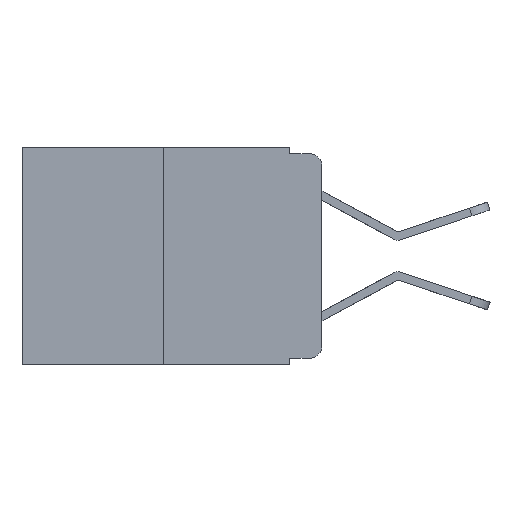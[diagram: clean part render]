
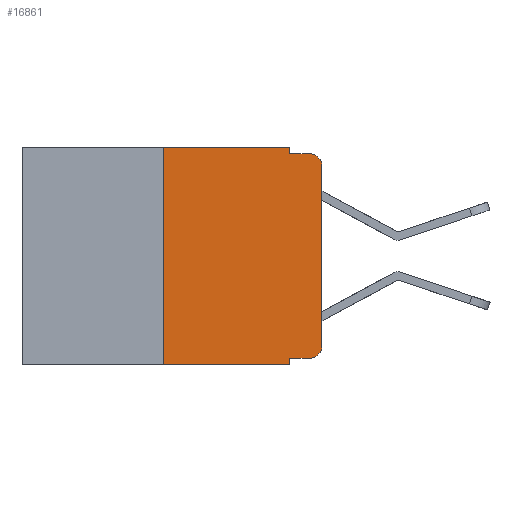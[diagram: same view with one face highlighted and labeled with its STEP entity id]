
A CAD part, left-side view. The second image highlights one B-rep face of the part: STEP entity #16861.
In plain terms, the highlighted planar face has unit normal (-1, 0, 0).
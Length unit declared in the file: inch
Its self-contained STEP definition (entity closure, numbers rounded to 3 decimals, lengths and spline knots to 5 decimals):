
#373 = DIRECTION ( 'NONE',  ( 0., 0., 1. ) ) ;
#494 = CARTESIAN_POINT ( 'NONE',  ( 0., 0.473, -0.343 ) ) ;
#852 = CARTESIAN_POINT ( 'NONE',  ( 0., 0.051, -0.01 ) ) ;
#1070 = EDGE_CURVE ( 'NONE', #14633, #12487, #20263, .T. ) ;
#1912 = LINE ( 'NONE', #2142, #10942 ) ;
#2142 = CARTESIAN_POINT ( 'NONE',  ( 0., 0.051, 0. ) ) ;
#2144 = CARTESIAN_POINT ( 'NONE',  ( 0., 0.25, -0.343 ) ) ;
#2176 = LINE ( 'NONE', #494, #15913 ) ;
#2320 = DIRECTION ( 'NONE',  ( 0., -1., 0. ) ) ;
#3552 = CARTESIAN_POINT ( 'NONE',  ( 0., 0.473, 0. ) ) ;
#3601 = ORIENTED_EDGE ( 'NONE', *, *, #10700, .F. ) ;
#3766 = EDGE_CURVE ( 'NONE', #4476, #6457, #15934, .T. ) ;
#4034 = CARTESIAN_POINT ( 'NONE',  ( 0., 0.02, -0.333 ) ) ;
#4049 = ORIENTED_EDGE ( 'NONE', *, *, #1070, .T. ) ;
#4253 = VERTEX_POINT ( 'NONE', #15675 ) ;
#4284 = LINE ( 'NONE', #21604, #13977 ) ;
#4476 = VERTEX_POINT ( 'NONE', #15097 ) ;
#5016 = VERTEX_POINT ( 'NONE', #8827 ) ;
#5936 = DIRECTION ( 'NONE',  ( 0., 0., -1. ) ) ;
#6019 = EDGE_CURVE ( 'NONE', #13148, #22199, #1912, .T. ) ;
#6223 = DIRECTION ( 'NONE',  ( 0., -1., 0. ) ) ;
#6457 = VERTEX_POINT ( 'NONE', #4034 ) ;
#6621 = VECTOR ( 'NONE', #19527, 39.37008 ) ;
#6659 = ORIENTED_EDGE ( 'NONE', *, *, #11068, .F. ) ;
#7290 = LINE ( 'NONE', #19115, #19686 ) ;
#7322 = VERTEX_POINT ( 'NONE', #2144 ) ;
#7634 = DIRECTION ( 'NONE',  ( 0., 0., -1. ) ) ;
#7727 = CARTESIAN_POINT ( 'NONE',  ( 0., 0.02, -0.03 ) ) ;
#7771 = AXIS2_PLACEMENT_3D ( 'NONE', #18124, #19796, #7634 ) ;
#7900 = VECTOR ( 'NONE', #373, 39.37008 ) ;
#8179 = EDGE_CURVE ( 'NONE', #6457, #5016, #16416, .T. ) ;
#8603 = ORIENTED_EDGE ( 'NONE', *, *, #8179, .T. ) ;
#8810 = ORIENTED_EDGE ( 'NONE', *, *, #17277, .T. ) ;
#8827 = CARTESIAN_POINT ( 'NONE',  ( 0., 0., -0.313 ) ) ;
#8864 = DIRECTION ( 'NONE',  ( 0., 0., 1. ) ) ;
#8943 = VECTOR ( 'NONE', #2320, 39.37008 ) ;
#9065 = DIRECTION ( 'NONE',  ( 1., 0., 0. ) ) ;
#9203 = DIRECTION ( 'NONE',  ( -1., 0., 0. ) ) ;
#10571 = AXIS2_PLACEMENT_3D ( 'NONE', #7727, #9203, #5936 ) ;
#10700 = EDGE_CURVE ( 'NONE', #4476, #4253, #4284, .T. ) ;
#10942 = VECTOR ( 'NONE', #14406, 39.37008 ) ;
#11068 = EDGE_CURVE ( 'NONE', #7322, #12865, #7290, .T. ) ;
#11308 = CARTESIAN_POINT ( 'NONE',  ( 0., 0.473, 0. ) ) ;
#12221 = EDGE_CURVE ( 'NONE', #22199, #12487, #16288, .T. ) ;
#12487 = VERTEX_POINT ( 'NONE', #12873 ) ;
#12562 = AXIS2_PLACEMENT_3D ( 'NONE', #3552, #9065, #21113 ) ;
#12716 = DIRECTION ( 'NONE',  ( 0., 0., -1. ) ) ;
#12865 = VERTEX_POINT ( 'NONE', #21071 ) ;
#12873 = CARTESIAN_POINT ( 'NONE',  ( 0., 0.02, -0.01 ) ) ;
#12923 = ORIENTED_EDGE ( 'NONE', *, *, #6019, .F. ) ;
#13148 = VERTEX_POINT ( 'NONE', #22019 ) ;
#13977 = VECTOR ( 'NONE', #12716, 39.37008 ) ;
#14020 = PLANE ( 'NONE',  #12562 ) ;
#14124 = CARTESIAN_POINT ( 'NONE',  ( 0., 0.051, -0.333 ) ) ;
#14170 = EDGE_LOOP ( 'NONE', ( #8810, #4049, #17989, #12923, #16042, #6659, #21036, #3601, #20827, #8603 ) ) ;
#14353 = FACE_OUTER_BOUND ( 'NONE', #14170, .T. ) ;
#14406 = DIRECTION ( 'NONE',  ( 0., 0., -1. ) ) ;
#14633 = VERTEX_POINT ( 'NONE', #16102 ) ;
#15097 = CARTESIAN_POINT ( 'NONE',  ( 0., 0.051, -0.333 ) ) ;
#15168 = CARTESIAN_POINT ( 'NONE',  ( 0., 0.051, -0.01 ) ) ;
#15675 = CARTESIAN_POINT ( 'NONE',  ( 0., 0.051, -0.343 ) ) ;
#15803 = LINE ( 'NONE', #21085, #7900 ) ;
#15913 = VECTOR ( 'NONE', #21203, 39.37008 ) ;
#15934 = LINE ( 'NONE', #14124, #6621 ) ;
#16042 = ORIENTED_EDGE ( 'NONE', *, *, #21222, .F. ) ;
#16102 = CARTESIAN_POINT ( 'NONE',  ( 0., 0., -0.03 ) ) ;
#16288 = LINE ( 'NONE', #852, #8943 ) ;
#16416 = CIRCLE ( 'NONE', #7771, 0.02 ) ;
#16861 = ADVANCED_FACE ( 'NONE', ( #14353 ), #14020, .F. ) ;
#17277 = EDGE_CURVE ( 'NONE', #5016, #14633, #15803, .T. ) ;
#17989 = ORIENTED_EDGE ( 'NONE', *, *, #12221, .F. ) ;
#18124 = CARTESIAN_POINT ( 'NONE',  ( 0., 0.02, -0.313 ) ) ;
#19115 = CARTESIAN_POINT ( 'NONE',  ( 0., 0.25, 0. ) ) ;
#19527 = DIRECTION ( 'NONE',  ( 0., -1., 0. ) ) ;
#19686 = VECTOR ( 'NONE', #8864, 39.37008 ) ;
#19739 = LINE ( 'NONE', #11308, #20218 ) ;
#19796 = DIRECTION ( 'NONE',  ( -1., 0., 0. ) ) ;
#20218 = VECTOR ( 'NONE', #6223, 39.37008 ) ;
#20263 = CIRCLE ( 'NONE', #10571, 0.02 ) ;
#20827 = ORIENTED_EDGE ( 'NONE', *, *, #3766, .T. ) ;
#21019 = EDGE_CURVE ( 'NONE', #7322, #4253, #2176, .T. ) ;
#21036 = ORIENTED_EDGE ( 'NONE', *, *, #21019, .T. ) ;
#21071 = CARTESIAN_POINT ( 'NONE',  ( 0., 0.25, 0. ) ) ;
#21085 = CARTESIAN_POINT ( 'NONE',  ( 0., 0., 0. ) ) ;
#21113 = DIRECTION ( 'NONE',  ( 0., 0., -1. ) ) ;
#21203 = DIRECTION ( 'NONE',  ( 0., -1., 0. ) ) ;
#21222 = EDGE_CURVE ( 'NONE', #12865, #13148, #19739, .T. ) ;
#21604 = CARTESIAN_POINT ( 'NONE',  ( 0., 0.051, 0. ) ) ;
#22019 = CARTESIAN_POINT ( 'NONE',  ( 0., 0.051, 0. ) ) ;
#22199 = VERTEX_POINT ( 'NONE', #15168 ) ;
